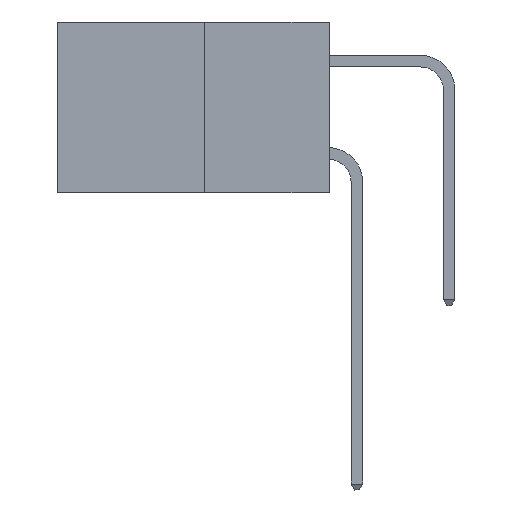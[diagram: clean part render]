
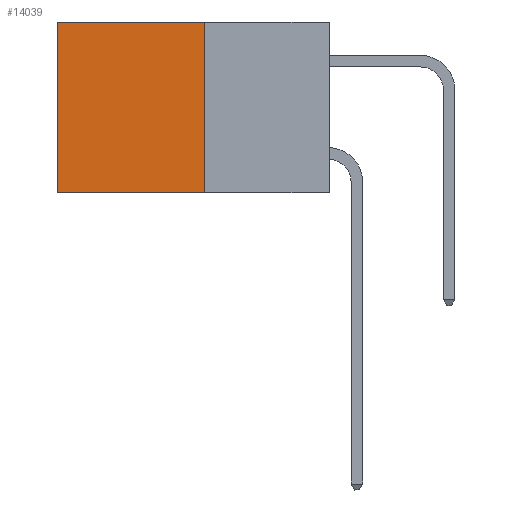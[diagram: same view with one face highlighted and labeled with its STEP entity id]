
A CAD part, left-side view. The second image highlights one B-rep face of the part: STEP entity #14039.
In plain terms, the highlighted planar face has unit normal (-1, 0, 0).
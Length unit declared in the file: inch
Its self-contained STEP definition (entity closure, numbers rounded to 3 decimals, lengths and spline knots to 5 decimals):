
#183 = ORIENTED_EDGE ( 'NONE', *, *, #20695, .T. ) ;
#436 = EDGE_LOOP ( 'NONE', ( #183, #12583, #20535, #19509 ) ) ;
#503 = CARTESIAN_POINT ( 'NONE',  ( 0.277, 0.27, 0. ) ) ;
#2119 = VECTOR ( 'NONE', #7425, 39.37008 ) ;
#5180 = CARTESIAN_POINT ( 'NONE',  ( 0.277, 0.59, -0.37 ) ) ;
#5210 = VERTEX_POINT ( 'NONE', #26378 ) ;
#5314 = CARTESIAN_POINT ( 'NONE',  ( 0.277, 0.27, -0.37 ) ) ;
#6041 = CARTESIAN_POINT ( 'NONE',  ( 0.277, 0.27, -0.37 ) ) ;
#7425 = DIRECTION ( 'NONE',  ( 0., 0., -1. ) ) ;
#7485 = CARTESIAN_POINT ( 'NONE',  ( 0.277, 0.59, -0.37 ) ) ;
#7611 = VECTOR ( 'NONE', #26881, 39.37008 ) ;
#8220 = LINE ( 'NONE', #5314, #13454 ) ;
#8284 = DIRECTION ( 'NONE',  ( 0., 0., -1. ) ) ;
#10071 = AXIS2_PLACEMENT_3D ( 'NONE', #6041, #21510, #8284 ) ;
#11029 = LINE ( 'NONE', #23143, #11709 ) ;
#11709 = VECTOR ( 'NONE', #12139, 39.37008 ) ;
#12139 = DIRECTION ( 'NONE',  ( 0., 0., -1. ) ) ;
#12505 = EDGE_CURVE ( 'NONE', #20408, #25097, #8220, .T. ) ;
#12583 = ORIENTED_EDGE ( 'NONE', *, *, #12505, .F. ) ;
#13454 = VECTOR ( 'NONE', #14203, 39.37008 ) ;
#13549 = LINE ( 'NONE', #503, #7611 ) ;
#13981 = CARTESIAN_POINT ( 'NONE',  ( 0.277, 0.59, 0. ) ) ;
#14039 = ADVANCED_FACE ( 'NONE', ( #26519 ), #19298, .F. ) ;
#14203 = DIRECTION ( 'NONE',  ( 0., 1., 0. ) ) ;
#19244 = CARTESIAN_POINT ( 'NONE',  ( 0.277, 0.27, -0.37 ) ) ;
#19298 = PLANE ( 'NONE',  #10071 ) ;
#19509 = ORIENTED_EDGE ( 'NONE', *, *, #22317, .T. ) ;
#20408 = VERTEX_POINT ( 'NONE', #19244 ) ;
#20535 = ORIENTED_EDGE ( 'NONE', *, *, #27276, .F. ) ;
#20695 = EDGE_CURVE ( 'NONE', #25693, #25097, #25508, .T. ) ;
#21510 = DIRECTION ( 'NONE',  ( 1., 0., 0. ) ) ;
#22317 = EDGE_CURVE ( 'NONE', #5210, #25693, #13549, .T. ) ;
#23143 = CARTESIAN_POINT ( 'NONE',  ( 0.277, 0.27, -0.37 ) ) ;
#25097 = VERTEX_POINT ( 'NONE', #7485 ) ;
#25508 = LINE ( 'NONE', #5180, #2119 ) ;
#25693 = VERTEX_POINT ( 'NONE', #13981 ) ;
#26378 = CARTESIAN_POINT ( 'NONE',  ( 0.277, 0.27, 0. ) ) ;
#26519 = FACE_OUTER_BOUND ( 'NONE', #436, .T. ) ;
#26881 = DIRECTION ( 'NONE',  ( 0., 1., 0. ) ) ;
#27276 = EDGE_CURVE ( 'NONE', #5210, #20408, #11029, .T. ) ;
